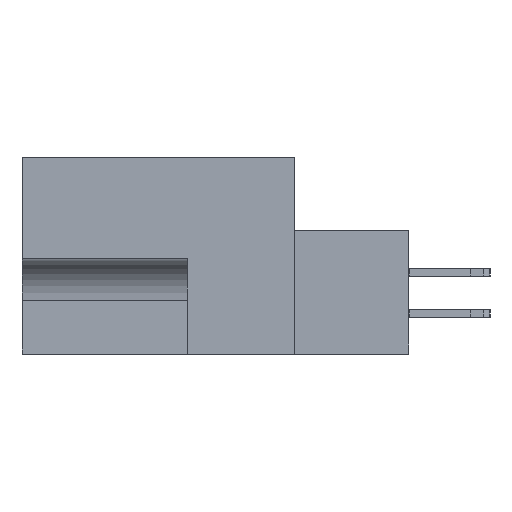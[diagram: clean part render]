
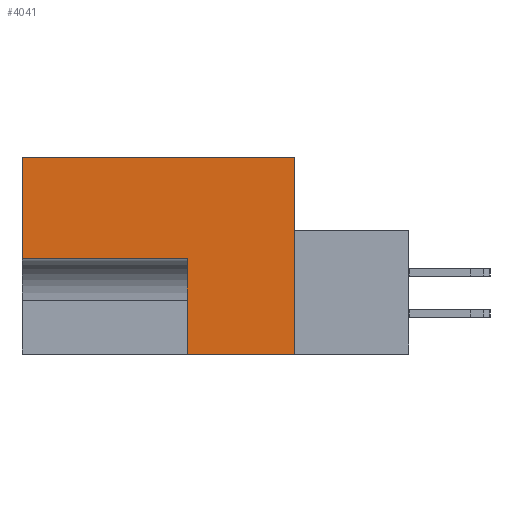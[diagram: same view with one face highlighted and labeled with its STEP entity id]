
A CAD part, left-side view. The second image highlights one B-rep face of the part: STEP entity #4041.
In plain terms, the highlighted planar face has unit normal (-1, 0, 0).
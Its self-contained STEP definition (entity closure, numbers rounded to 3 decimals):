
#245 = VECTOR ( 'NONE', #3769, 1000. ) ;
#430 = DIRECTION ( 'NONE',  ( 0., 0., -1. ) ) ;
#1788 = VECTOR ( 'NONE', #430, 1000. ) ;
#1893 = CARTESIAN_POINT ( 'NONE',  ( 0., 8.255, -15.088 ) ) ;
#2568 = DIRECTION ( 'NONE',  ( 0., 0., 1. ) ) ;
#3208 = DIRECTION ( 'NONE',  ( 0., 0., -1. ) ) ;
#3769 = DIRECTION ( 'NONE',  ( 0., 1., 0. ) ) ;
#4041 = ADVANCED_FACE ( 'NONE', ( #21675 ), #39108, .F. ) ;
#4541 = DIRECTION ( 'NONE',  ( 0., 0., 1. ) ) ;
#5309 = ORIENTED_EDGE ( 'NONE', *, *, #12948, .F. ) ;
#5516 = CARTESIAN_POINT ( 'NONE',  ( 0., 20.955, 0. ) ) ;
#6750 = CARTESIAN_POINT ( 'NONE',  ( 0., 20.955, -7.772 ) ) ;
#6928 = AXIS2_PLACEMENT_3D ( 'NONE', #43297, #27220, #3208 ) ;
#7296 = LINE ( 'NONE', #24857, #22900 ) ;
#10291 = DIRECTION ( 'NONE',  ( 0., 1., 0. ) ) ;
#11384 = EDGE_CURVE ( 'NONE', #35169, #51971, #37457, .T. ) ;
#12948 = EDGE_CURVE ( 'NONE', #37282, #39234, #32306, .T. ) ;
#15654 = VECTOR ( 'NONE', #2568, 1000. ) ;
#16643 = ORIENTED_EDGE ( 'NONE', *, *, #36547, .F. ) ;
#17096 = ORIENTED_EDGE ( 'NONE', *, *, #29313, .F. ) ;
#19179 = CARTESIAN_POINT ( 'NONE',  ( 0., 11.506, 0. ) ) ;
#20032 = LINE ( 'NONE', #1893, #15654 ) ;
#21675 = FACE_OUTER_BOUND ( 'NONE', #25586, .T. ) ;
#22900 = VECTOR ( 'NONE', #4541, 1000. ) ;
#23121 = LINE ( 'NONE', #32847, #1788 ) ;
#23759 = CARTESIAN_POINT ( 'NONE',  ( 0., 8.255, -7.772 ) ) ;
#24384 = EDGE_CURVE ( 'NONE', #51117, #35169, #7296, .T. ) ;
#24857 = CARTESIAN_POINT ( 'NONE',  ( 0., 20.955, -15.088 ) ) ;
#25437 = VECTOR ( 'NONE', #10291, 1000. ) ;
#25586 = EDGE_LOOP ( 'NONE', ( #5309, #17096, #48757, #38020, #16643, #46700 ) ) ;
#27220 = DIRECTION ( 'NONE',  ( 1., 0., 0. ) ) ;
#28964 = EDGE_CURVE ( 'NONE', #39234, #41304, #20032, .T. ) ;
#29313 = EDGE_CURVE ( 'NONE', #51971, #37282, #23121, .T. ) ;
#29711 = LINE ( 'NONE', #23759, #245 ) ;
#31806 = VECTOR ( 'NONE', #47187, 1000. ) ;
#32306 = LINE ( 'NONE', #34229, #25437 ) ;
#32847 = CARTESIAN_POINT ( 'NONE',  ( 0., 0., 0. ) ) ;
#34229 = CARTESIAN_POINT ( 'NONE',  ( 0., -8.814, -15.088 ) ) ;
#35169 = VERTEX_POINT ( 'NONE', #5516 ) ;
#36547 = EDGE_CURVE ( 'NONE', #41304, #51117, #29711, .T. ) ;
#37282 = VERTEX_POINT ( 'NONE', #46491 ) ;
#37457 = LINE ( 'NONE', #19179, #31806 ) ;
#38020 = ORIENTED_EDGE ( 'NONE', *, *, #24384, .F. ) ;
#39108 = PLANE ( 'NONE',  #6928 ) ;
#39234 = VERTEX_POINT ( 'NONE', #49627 ) ;
#40957 = CARTESIAN_POINT ( 'NONE',  ( 0., 8.255, -7.772 ) ) ;
#41304 = VERTEX_POINT ( 'NONE', #40957 ) ;
#43297 = CARTESIAN_POINT ( 'NONE',  ( 0., 0., 0. ) ) ;
#46491 = CARTESIAN_POINT ( 'NONE',  ( 0., 0., -15.088 ) ) ;
#46700 = ORIENTED_EDGE ( 'NONE', *, *, #28964, .F. ) ;
#47187 = DIRECTION ( 'NONE',  ( 0., -1., 0. ) ) ;
#48757 = ORIENTED_EDGE ( 'NONE', *, *, #11384, .F. ) ;
#49192 = CARTESIAN_POINT ( 'NONE',  ( 0., 0., 0. ) ) ;
#49627 = CARTESIAN_POINT ( 'NONE',  ( 0., 8.255, -15.088 ) ) ;
#51117 = VERTEX_POINT ( 'NONE', #6750 ) ;
#51971 = VERTEX_POINT ( 'NONE', #49192 ) ;
